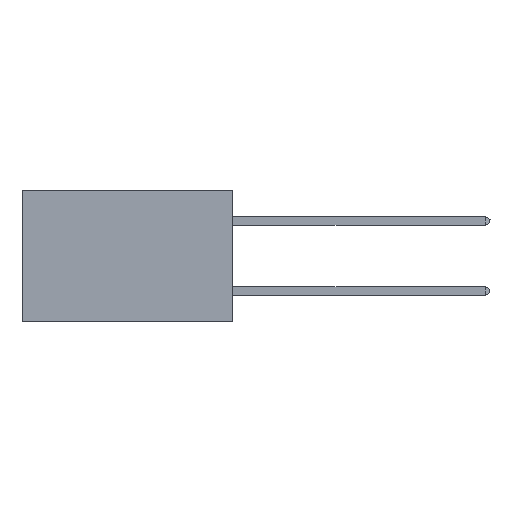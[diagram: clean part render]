
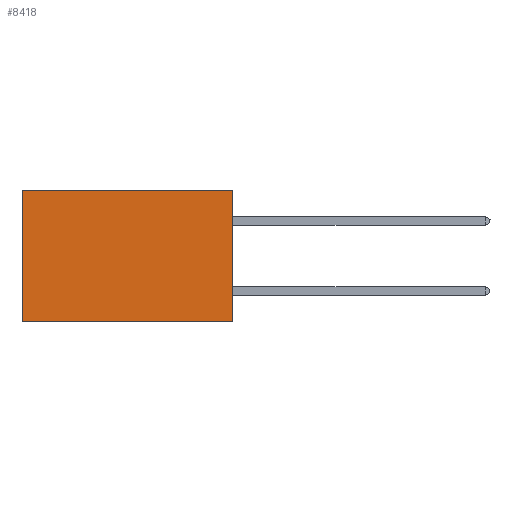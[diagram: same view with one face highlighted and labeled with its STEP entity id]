
A CAD part, left-side view. The second image highlights one B-rep face of the part: STEP entity #8418.
In plain terms, the highlighted planar face has unit normal (-1, 0, 0).
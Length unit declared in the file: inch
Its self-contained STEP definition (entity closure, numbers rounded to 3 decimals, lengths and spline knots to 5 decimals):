
#197 = VERTEX_POINT ( 'NONE', #11304 ) ;
#202 = LINE ( 'NONE', #6426, #10423 ) ;
#1106 = FACE_OUTER_BOUND ( 'NONE', #9552, .T. ) ;
#1655 = LINE ( 'NONE', #5816, #12825 ) ;
#1693 = LINE ( 'NONE', #12878, #4862 ) ;
#2068 = ORIENTED_EDGE ( 'NONE', *, *, #5518, .T. ) ;
#2112 = PLANE ( 'NONE',  #10261 ) ;
#3709 = DIRECTION ( 'NONE',  ( 0., 0., -1. ) ) ;
#3790 = DIRECTION ( 'NONE',  ( 0., 0., -1. ) ) ;
#3864 = EDGE_CURVE ( 'NONE', #5211, #10169, #4863, .T. ) ;
#4058 = CARTESIAN_POINT ( 'NONE',  ( 0.2875, 0., 0. ) ) ;
#4190 = DIRECTION ( 'NONE',  ( 1., 0., 0. ) ) ;
#4200 = ORIENTED_EDGE ( 'NONE', *, *, #7509, .T. ) ;
#4862 = VECTOR ( 'NONE', #3709, 39.37008 ) ;
#4863 = LINE ( 'NONE', #7675, #11061 ) ;
#5211 = VERTEX_POINT ( 'NONE', #4058 ) ;
#5518 = EDGE_CURVE ( 'NONE', #5767, #197, #1693, .T. ) ;
#5767 = VERTEX_POINT ( 'NONE', #10576 ) ;
#5816 = CARTESIAN_POINT ( 'NONE',  ( 0.2875, 0., -0.375 ) ) ;
#6331 = CARTESIAN_POINT ( 'NONE',  ( 0.2875, 0., -0.375 ) ) ;
#6426 = CARTESIAN_POINT ( 'NONE',  ( 0.2875, 0., 0. ) ) ;
#7243 = ORIENTED_EDGE ( 'NONE', *, *, #11312, .F. ) ;
#7509 = EDGE_CURVE ( 'NONE', #5211, #5767, #202, .T. ) ;
#7675 = CARTESIAN_POINT ( 'NONE',  ( 0.2875, 0., -0.375 ) ) ;
#7945 = DIRECTION ( 'NONE',  ( 0., 1., 0. ) ) ;
#8272 = CARTESIAN_POINT ( 'NONE',  ( 0.2875, 0., -0.375 ) ) ;
#8418 = ADVANCED_FACE ( 'NONE', ( #1106 ), #2112, .F. ) ;
#9552 = EDGE_LOOP ( 'NONE', ( #2068, #7243, #9575, #4200 ) ) ;
#9575 = ORIENTED_EDGE ( 'NONE', *, *, #3864, .F. ) ;
#10169 = VERTEX_POINT ( 'NONE', #6331 ) ;
#10261 = AXIS2_PLACEMENT_3D ( 'NONE', #8272, #4190, #11340 ) ;
#10423 = VECTOR ( 'NONE', #12645, 39.37008 ) ;
#10576 = CARTESIAN_POINT ( 'NONE',  ( 0.2875, 0.6, 0. ) ) ;
#11061 = VECTOR ( 'NONE', #3790, 39.37008 ) ;
#11304 = CARTESIAN_POINT ( 'NONE',  ( 0.2875, 0.6, -0.375 ) ) ;
#11312 = EDGE_CURVE ( 'NONE', #10169, #197, #1655, .T. ) ;
#11340 = DIRECTION ( 'NONE',  ( 0., 0., -1. ) ) ;
#12645 = DIRECTION ( 'NONE',  ( 0., 1., 0. ) ) ;
#12825 = VECTOR ( 'NONE', #7945, 39.37008 ) ;
#12878 = CARTESIAN_POINT ( 'NONE',  ( 0.2875, 0.6, -0.375 ) ) ;
